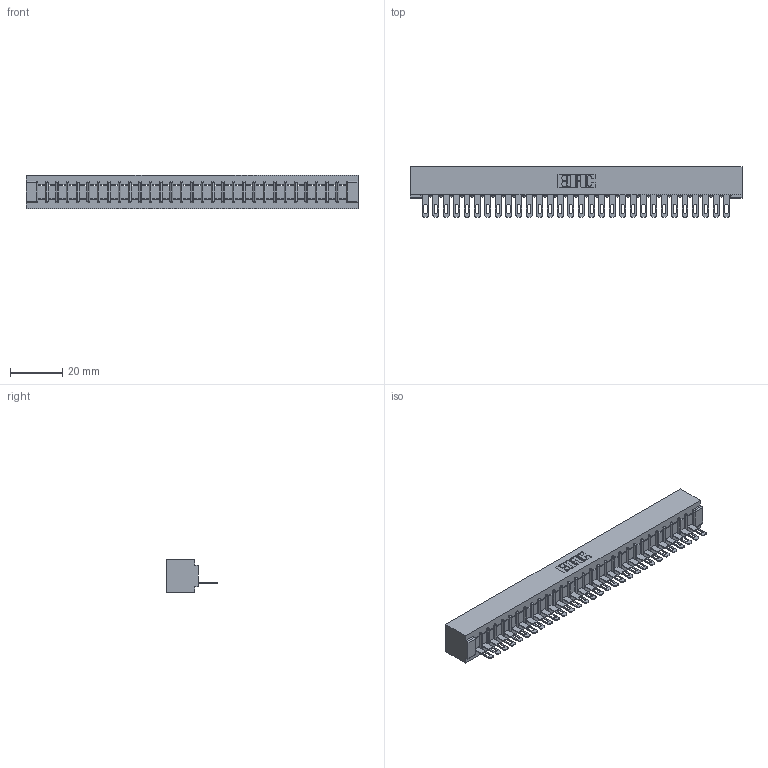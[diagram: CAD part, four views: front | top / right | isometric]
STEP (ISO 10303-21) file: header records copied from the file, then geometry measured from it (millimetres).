
FILE_DESCRIPTION (( 'STEP AP203' ), '1' );
FILE_NAME ('357-030-405-101.STEP', '2020-10-02T00:13:06', ( '' ), ( '' ), 'SwSTEP 2.0', 'SolidWorks 2020', '' );
FILE_SCHEMA (( 'CONFIG_CONTROL_DESIGN' ));
Length unit declared in the file: inch
Products named in the file (3): 357-030-405-101; 307-290-001_505; 307 Part_No Mounting Lugs
Assembly tree (31 placements, depth 2):
  357-030-405-101
    307 Part_No Mounting Lugs
    307-290-001_505  x30
Bounding box: 126.75 x 19.18 x 12.7 mm (x, y, z)
Volume: 13639.3 mm3; surface area: 14697.7 mm2
Topology: 31 solids, 31 shells, 1821 faces, 5159 edges, 3314 vertices
Faces by surface type: plane 1146, cylinder 613, sphere 62
Entity records: 26894 total; most frequent: CARTESIAN_POINT 4524, ORIENTED_EDGE 4510, DIRECTION 4407, EDGE_CURVE 2255, VECTOR 1725, LINE 1725, VERTEX_POINT 1458, AXIS2_PLACEMENT_3D 1341
